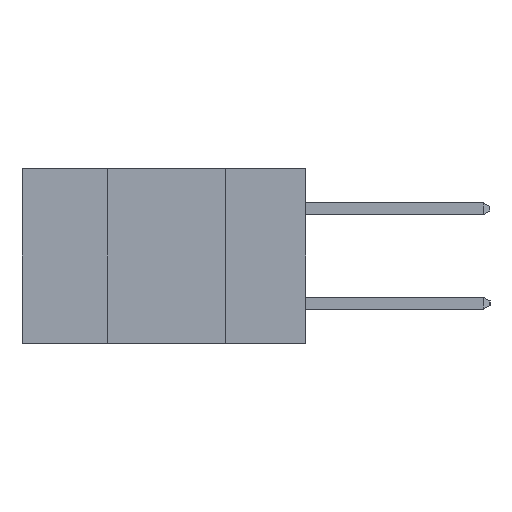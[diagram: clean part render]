
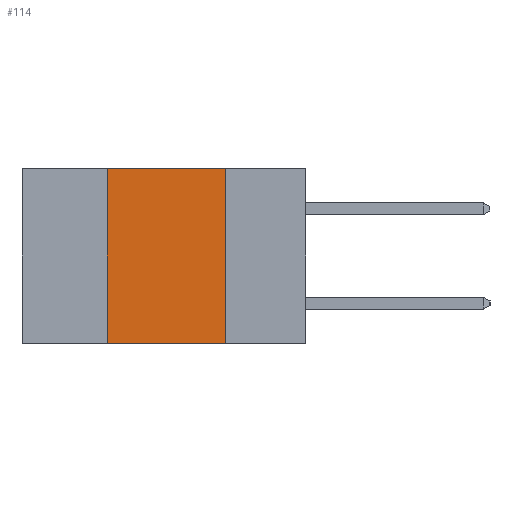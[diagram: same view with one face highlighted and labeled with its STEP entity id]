
A CAD part, left-side view. The second image highlights one B-rep face of the part: STEP entity #114.
In plain terms, the highlighted planar face has unit normal (-1, 0, 0).
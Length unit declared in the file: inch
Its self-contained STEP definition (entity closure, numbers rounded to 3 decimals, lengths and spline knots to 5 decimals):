
#114 = ADVANCED_FACE ( 'NONE', ( #6661 ), #2632, .F. ) ;
#214 = ORIENTED_EDGE ( 'NONE', *, *, #1473, .F. ) ;
#243 = CARTESIAN_POINT ( 'NONE',  ( 0., 0.6, 0. ) ) ;
#378 = DIRECTION ( 'NONE',  ( 0., -1., 0. ) ) ;
#648 = VERTEX_POINT ( 'NONE', #12415 ) ;
#666 = DIRECTION ( 'NONE',  ( 0., 0., -1. ) ) ;
#678 = DIRECTION ( 'NONE',  ( 1., 0., 0. ) ) ;
#1036 = DIRECTION ( 'NONE',  ( 0., 0., -1. ) ) ;
#1179 = VECTOR ( 'NONE', #378, 39.37008 ) ;
#1308 = CARTESIAN_POINT ( 'NONE',  ( 0., 0.17, -0.37 ) ) ;
#1473 = EDGE_CURVE ( 'NONE', #1851, #648, #4888, .T. ) ;
#1851 = VERTEX_POINT ( 'NONE', #9137 ) ;
#2306 = CARTESIAN_POINT ( 'NONE',  ( 0., 0.6, 0. ) ) ;
#2632 = PLANE ( 'NONE',  #3670 ) ;
#3210 = LINE ( 'NONE', #5578, #8502 ) ;
#3670 = AXIS2_PLACEMENT_3D ( 'NONE', #2306, #678, #666 ) ;
#4349 = VERTEX_POINT ( 'NONE', #8095 ) ;
#4869 = VERTEX_POINT ( 'NONE', #7952 ) ;
#4888 = LINE ( 'NONE', #10740, #7254 ) ;
#5544 = DIRECTION ( 'NONE',  ( 0., -1., 0. ) ) ;
#5578 = CARTESIAN_POINT ( 'NONE',  ( 0., 0.6, -0.37 ) ) ;
#6228 = ORIENTED_EDGE ( 'NONE', *, *, #12439, .T. ) ;
#6661 = FACE_OUTER_BOUND ( 'NONE', #11747, .T. ) ;
#6860 = VECTOR ( 'NONE', #1036, 39.37008 ) ;
#7254 = VECTOR ( 'NONE', #10726, 39.37008 ) ;
#7482 = LINE ( 'NONE', #1308, #6860 ) ;
#7936 = EDGE_CURVE ( 'NONE', #648, #4349, #11732, .T. ) ;
#7952 = CARTESIAN_POINT ( 'NONE',  ( 0., 0.17, -0.37 ) ) ;
#8095 = CARTESIAN_POINT ( 'NONE',  ( 0., 0.17, 0. ) ) ;
#8502 = VECTOR ( 'NONE', #5544, 39.37008 ) ;
#9137 = CARTESIAN_POINT ( 'NONE',  ( 0., 0.42, -0.37 ) ) ;
#10726 = DIRECTION ( 'NONE',  ( 0., 0., 1. ) ) ;
#10740 = CARTESIAN_POINT ( 'NONE',  ( 0., 0.42, -0.37 ) ) ;
#10925 = EDGE_CURVE ( 'NONE', #4349, #4869, #7482, .T. ) ;
#10956 = ORIENTED_EDGE ( 'NONE', *, *, #10925, .F. ) ;
#11732 = LINE ( 'NONE', #243, #1179 ) ;
#11747 = EDGE_LOOP ( 'NONE', ( #10956, #12136, #214, #6228 ) ) ;
#12136 = ORIENTED_EDGE ( 'NONE', *, *, #7936, .F. ) ;
#12415 = CARTESIAN_POINT ( 'NONE',  ( 0., 0.42, 0. ) ) ;
#12439 = EDGE_CURVE ( 'NONE', #1851, #4869, #3210, .T. ) ;
